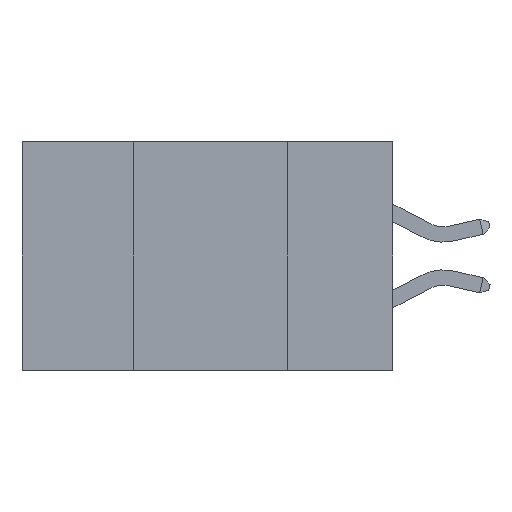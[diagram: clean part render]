
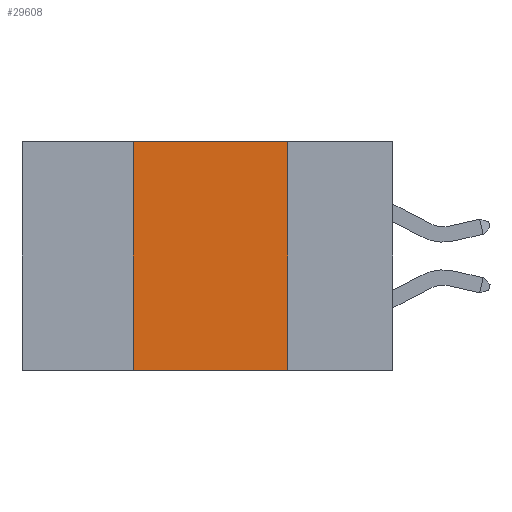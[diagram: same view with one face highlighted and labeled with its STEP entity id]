
A CAD part, left-side view. The second image highlights one B-rep face of the part: STEP entity #29608.
In plain terms, the highlighted planar face has unit normal (-1, 0, 0).
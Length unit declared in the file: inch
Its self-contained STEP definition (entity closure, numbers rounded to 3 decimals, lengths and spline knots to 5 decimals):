
#924 = VERTEX_POINT ( 'NONE', #1975 ) ;
#1451 = VECTOR ( 'NONE', #14034, 39.37008 ) ;
#1975 = CARTESIAN_POINT ( 'NONE',  ( 0., 0.17, 0. ) ) ;
#2235 = DIRECTION ( 'NONE',  ( 0., 0., -1. ) ) ;
#3286 = CARTESIAN_POINT ( 'NONE',  ( 0., 0.42, 0. ) ) ;
#4296 = EDGE_CURVE ( 'NONE', #6375, #924, #20427, .T. ) ;
#5159 = VERTEX_POINT ( 'NONE', #11726 ) ;
#6143 = LINE ( 'NONE', #7900, #23524 ) ;
#6375 = VERTEX_POINT ( 'NONE', #24822 ) ;
#6784 = ORIENTED_EDGE ( 'NONE', *, *, #19803, .F. ) ;
#7485 = DIRECTION ( 'NONE',  ( 0., -1., 0. ) ) ;
#7699 = CARTESIAN_POINT ( 'NONE',  ( 0., 0.6, -0.37 ) ) ;
#7900 = CARTESIAN_POINT ( 'NONE',  ( 0., 0.17, 0. ) ) ;
#9125 = ORIENTED_EDGE ( 'NONE', *, *, #23976, .F. ) ;
#9494 = CARTESIAN_POINT ( 'NONE',  ( 0., 0.6, 0. ) ) ;
#9625 = AXIS2_PLACEMENT_3D ( 'NONE', #9494, #22210, #2235 ) ;
#10153 = EDGE_LOOP ( 'NONE', ( #6784, #21063, #9125, #10202 ) ) ;
#10202 = ORIENTED_EDGE ( 'NONE', *, *, #21403, .T. ) ;
#11726 = CARTESIAN_POINT ( 'NONE',  ( 0., 0.42, -0.37 ) ) ;
#13179 = DIRECTION ( 'NONE',  ( 0., 0., -1. ) ) ;
#14034 = DIRECTION ( 'NONE',  ( 0., -1., 0. ) ) ;
#16287 = VECTOR ( 'NONE', #18268, 39.37008 ) ;
#16896 = PLANE ( 'NONE',  #9625 ) ;
#18268 = DIRECTION ( 'NONE',  ( 0., 0., 1. ) ) ;
#18665 = LINE ( 'NONE', #3286, #16287 ) ;
#19617 = CARTESIAN_POINT ( 'NONE',  ( 0., 0.17, -0.37 ) ) ;
#19803 = EDGE_CURVE ( 'NONE', #924, #22145, #6143, .T. ) ;
#20427 = LINE ( 'NONE', #26619, #1451 ) ;
#21063 = ORIENTED_EDGE ( 'NONE', *, *, #4296, .F. ) ;
#21403 = EDGE_CURVE ( 'NONE', #5159, #22145, #29522, .T. ) ;
#22145 = VERTEX_POINT ( 'NONE', #19617 ) ;
#22210 = DIRECTION ( 'NONE',  ( 1., 0., 0. ) ) ;
#22448 = VECTOR ( 'NONE', #7485, 39.37008 ) ;
#22967 = FACE_OUTER_BOUND ( 'NONE', #10153, .T. ) ;
#23524 = VECTOR ( 'NONE', #13179, 39.37008 ) ;
#23976 = EDGE_CURVE ( 'NONE', #5159, #6375, #18665, .T. ) ;
#24822 = CARTESIAN_POINT ( 'NONE',  ( 0., 0.42, 0. ) ) ;
#26619 = CARTESIAN_POINT ( 'NONE',  ( 0., 0.6, 0. ) ) ;
#29522 = LINE ( 'NONE', #7699, #22448 ) ;
#29608 = ADVANCED_FACE ( 'NONE', ( #22967 ), #16896, .F. ) ;
